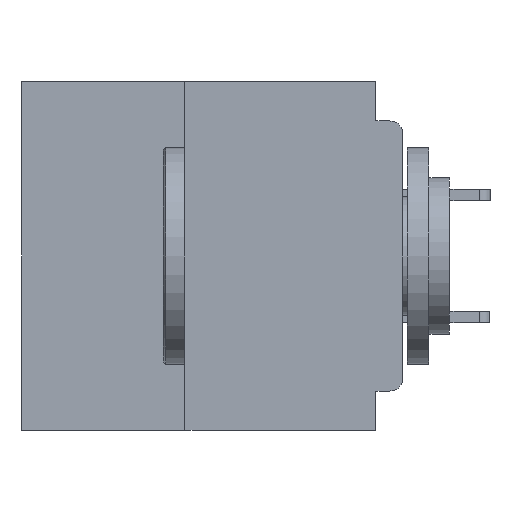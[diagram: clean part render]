
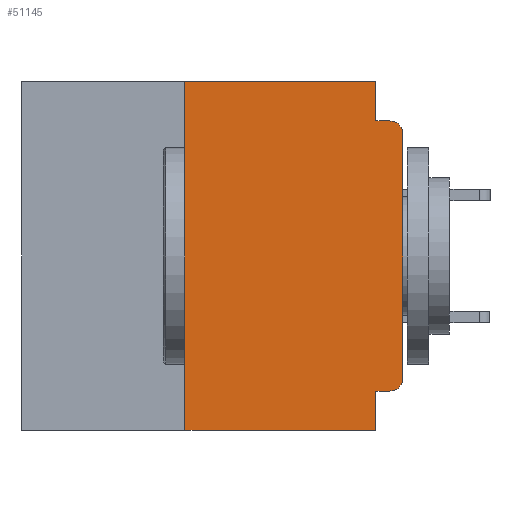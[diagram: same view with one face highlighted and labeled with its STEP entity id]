
A CAD part, left-side view. The second image highlights one B-rep face of the part: STEP entity #51145.
In plain terms, the highlighted planar face has unit normal (-1, 0, 0).
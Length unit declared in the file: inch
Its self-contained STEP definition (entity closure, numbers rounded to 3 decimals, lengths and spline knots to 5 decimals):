
#876 = CARTESIAN_POINT ( 'NONE',  ( 0., 0.437, -0.4 ) ) ;
#1055 = ORIENTED_EDGE ( 'NONE', *, *, #28160, .T. ) ;
#1147 = LINE ( 'NONE', #37851, #35743 ) ;
#1157 = DIRECTION ( 'NONE',  ( 0., -1., 0. ) ) ;
#1261 = CARTESIAN_POINT ( 'NONE',  ( 0., 0.015, -0.045 ) ) ;
#2275 = VECTOR ( 'NONE', #7678, 39.37008 ) ;
#3140 = CARTESIAN_POINT ( 'NONE',  ( 0., 0.031, 0. ) ) ;
#3490 = ORIENTED_EDGE ( 'NONE', *, *, #53068, .F. ) ;
#3738 = LINE ( 'NONE', #9857, #14346 ) ;
#3835 = LINE ( 'NONE', #52556, #25039 ) ;
#4348 = DIRECTION ( 'NONE',  ( 0., 0., -1. ) ) ;
#4718 = DIRECTION ( 'NONE',  ( -1., 0., 0. ) ) ;
#5723 = CARTESIAN_POINT ( 'NONE',  ( 0., 0., 0. ) ) ;
#6127 = CARTESIAN_POINT ( 'NONE',  ( 0., 0.25, 0. ) ) ;
#6750 = CARTESIAN_POINT ( 'NONE',  ( 0., 0.015, -0.34 ) ) ;
#7678 = DIRECTION ( 'NONE',  ( 0., 0., -1. ) ) ;
#7839 = CARTESIAN_POINT ( 'NONE',  ( 0., 0.25, -0.4 ) ) ;
#9857 = CARTESIAN_POINT ( 'NONE',  ( 0., 0., -0.355 ) ) ;
#10209 = CARTESIAN_POINT ( 'NONE',  ( 0., 0.031, 0. ) ) ;
#10392 = VERTEX_POINT ( 'NONE', #1261 ) ;
#11238 = DIRECTION ( 'NONE',  ( 0., 0., -1. ) ) ;
#11470 = VECTOR ( 'NONE', #37317, 39.37008 ) ;
#11910 = VERTEX_POINT ( 'NONE', #44276 ) ;
#12202 = AXIS2_PLACEMENT_3D ( 'NONE', #6750, #38312, #11238 ) ;
#14346 = VECTOR ( 'NONE', #14422, 39.37008 ) ;
#14422 = DIRECTION ( 'NONE',  ( 0., 1., 0. ) ) ;
#14561 = CARTESIAN_POINT ( 'NONE',  ( 0., 0., -0.045 ) ) ;
#14858 = CARTESIAN_POINT ( 'NONE',  ( 0., 0.015, -0.355 ) ) ;
#14944 = EDGE_CURVE ( 'NONE', #34987, #16887, #1147, .T. ) ;
#15818 = EDGE_CURVE ( 'NONE', #16887, #37806, #3835, .T. ) ;
#16497 = DIRECTION ( 'NONE',  ( 0., -1., 0. ) ) ;
#16887 = VERTEX_POINT ( 'NONE', #6127 ) ;
#17088 = EDGE_CURVE ( 'NONE', #37806, #46285, #38270, .T. ) ;
#17561 = VERTEX_POINT ( 'NONE', #29739 ) ;
#17769 = PLANE ( 'NONE',  #57338 ) ;
#19627 = EDGE_CURVE ( 'NONE', #34987, #11910, #21036, .T. ) ;
#19703 = DIRECTION ( 'NONE',  ( 0., 0., 1. ) ) ;
#21036 = LINE ( 'NONE', #876, #55565 ) ;
#21214 = ORIENTED_EDGE ( 'NONE', *, *, #55636, .T. ) ;
#23377 = DIRECTION ( 'NONE',  ( 0., -1., 0. ) ) ;
#23524 = LINE ( 'NONE', #5723, #11470 ) ;
#23735 = VERTEX_POINT ( 'NONE', #14858 ) ;
#25039 = VECTOR ( 'NONE', #16497, 39.37008 ) ;
#28160 = EDGE_CURVE ( 'NONE', #28590, #10392, #52051, .T. ) ;
#28590 = VERTEX_POINT ( 'NONE', #43713 ) ;
#29626 = DIRECTION ( 'NONE',  ( 0., 0., -1. ) ) ;
#29739 = CARTESIAN_POINT ( 'NONE',  ( 0., 0.031, -0.355 ) ) ;
#30677 = EDGE_CURVE ( 'NONE', #17561, #11910, #47474, .T. ) ;
#31385 = DIRECTION ( 'NONE',  ( 1., 0., 0. ) ) ;
#31749 = CARTESIAN_POINT ( 'NONE',  ( 0., 0.015, -0.06 ) ) ;
#33746 = ORIENTED_EDGE ( 'NONE', *, *, #19627, .T. ) ;
#34987 = VERTEX_POINT ( 'NONE', #7839 ) ;
#35743 = VECTOR ( 'NONE', #19703, 39.37008 ) ;
#35751 = CARTESIAN_POINT ( 'NONE',  ( 0., 0.437, 0. ) ) ;
#35814 = VECTOR ( 'NONE', #1157, 39.37008 ) ;
#36315 = DIRECTION ( 'NONE',  ( 0., 0., -1. ) ) ;
#36484 = ORIENTED_EDGE ( 'NONE', *, *, #53111, .T. ) ;
#37317 = DIRECTION ( 'NONE',  ( 0., 0., 1. ) ) ;
#37510 = CARTESIAN_POINT ( 'NONE',  ( 0., 0.031, -0.045 ) ) ;
#37806 = VERTEX_POINT ( 'NONE', #10209 ) ;
#37851 = CARTESIAN_POINT ( 'NONE',  ( 0., 0.25, -0.4 ) ) ;
#38270 = LINE ( 'NONE', #3140, #2275 ) ;
#38312 = DIRECTION ( 'NONE',  ( -1., 0., 0. ) ) ;
#38860 = AXIS2_PLACEMENT_3D ( 'NONE', #31749, #4718, #36315 ) ;
#40621 = EDGE_LOOP ( 'NONE', ( #36484, #1055, #57967, #43762, #49913, #54675, #33746, #50608, #3490, #21214 ) ) ;
#41825 = EDGE_CURVE ( 'NONE', #46285, #10392, #49190, .T. ) ;
#42803 = CIRCLE ( 'NONE', #12202, 0.015 ) ;
#43713 = CARTESIAN_POINT ( 'NONE',  ( 0., 0., -0.06 ) ) ;
#43762 = ORIENTED_EDGE ( 'NONE', *, *, #17088, .F. ) ;
#44198 = FACE_OUTER_BOUND ( 'NONE', #40621, .T. ) ;
#44276 = CARTESIAN_POINT ( 'NONE',  ( 0., 0.031, -0.4 ) ) ;
#46061 = VECTOR ( 'NONE', #29626, 39.37008 ) ;
#46285 = VERTEX_POINT ( 'NONE', #37510 ) ;
#46803 = VERTEX_POINT ( 'NONE', #54550 ) ;
#47474 = LINE ( 'NONE', #52076, #46061 ) ;
#49190 = LINE ( 'NONE', #14561, #35814 ) ;
#49913 = ORIENTED_EDGE ( 'NONE', *, *, #15818, .F. ) ;
#50608 = ORIENTED_EDGE ( 'NONE', *, *, #30677, .F. ) ;
#51145 = ADVANCED_FACE ( 'NONE', ( #44198 ), #17769, .F. ) ;
#52051 = CIRCLE ( 'NONE', #38860, 0.015 ) ;
#52076 = CARTESIAN_POINT ( 'NONE',  ( 0., 0.031, -0.4 ) ) ;
#52556 = CARTESIAN_POINT ( 'NONE',  ( 0., 0.437, 0. ) ) ;
#53068 = EDGE_CURVE ( 'NONE', #23735, #17561, #3738, .T. ) ;
#53111 = EDGE_CURVE ( 'NONE', #46803, #28590, #23524, .T. ) ;
#54550 = CARTESIAN_POINT ( 'NONE',  ( 0., 0., -0.34 ) ) ;
#54675 = ORIENTED_EDGE ( 'NONE', *, *, #14944, .F. ) ;
#55565 = VECTOR ( 'NONE', #23377, 39.37008 ) ;
#55636 = EDGE_CURVE ( 'NONE', #23735, #46803, #42803, .T. ) ;
#57338 = AXIS2_PLACEMENT_3D ( 'NONE', #35751, #31385, #4348 ) ;
#57967 = ORIENTED_EDGE ( 'NONE', *, *, #41825, .F. ) ;
